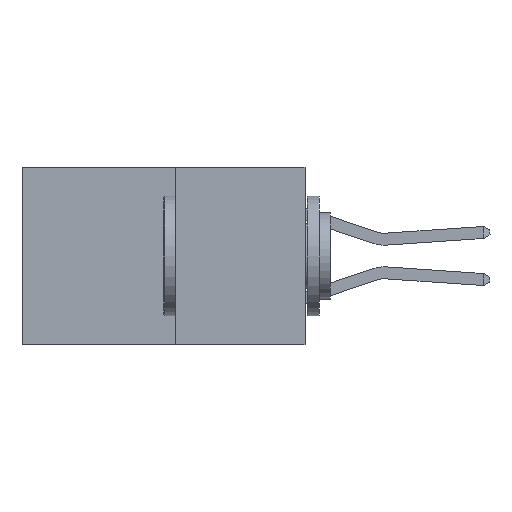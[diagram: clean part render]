
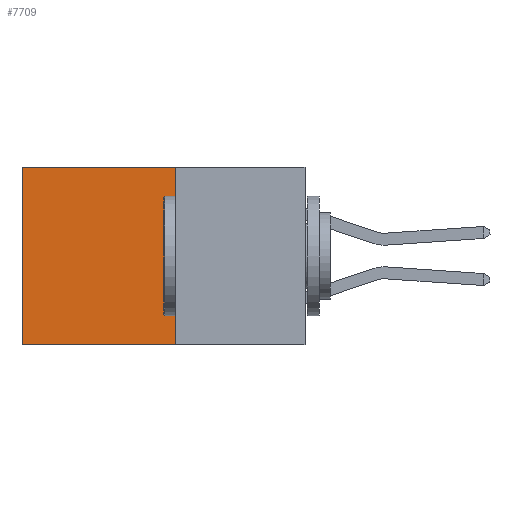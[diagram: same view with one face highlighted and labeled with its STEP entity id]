
A CAD part, left-side view. The second image highlights one B-rep face of the part: STEP entity #7709.
In plain terms, the highlighted planar face has unit normal (-1, 0, 0).
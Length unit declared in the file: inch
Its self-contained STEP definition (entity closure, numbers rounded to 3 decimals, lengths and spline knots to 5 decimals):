
#65 = CARTESIAN_POINT ( 'NONE',  ( 0.277, 0.27, 0. ) ) ;
#237 = VECTOR ( 'NONE', #8344, 39.37008 ) ;
#257 = EDGE_CURVE ( 'NONE', #1255, #6947, #2991, .T. ) ;
#728 = EDGE_CURVE ( 'NONE', #9189, #6947, #5139, .T. ) ;
#938 = DIRECTION ( 'NONE',  ( 0., 1., 0. ) ) ;
#1255 = VERTEX_POINT ( 'NONE', #4442 ) ;
#1571 = ORIENTED_EDGE ( 'NONE', *, *, #3591, .F. ) ;
#1621 = CARTESIAN_POINT ( 'NONE',  ( 0.277, 0.59, -0.37 ) ) ;
#1631 = AXIS2_PLACEMENT_3D ( 'NONE', #5844, #7537, #2435 ) ;
#1643 = CARTESIAN_POINT ( 'NONE',  ( 0.277, 0.27, -0.37 ) ) ;
#2001 = CARTESIAN_POINT ( 'NONE',  ( 0.277, 0.27, 0. ) ) ;
#2435 = DIRECTION ( 'NONE',  ( 0., 0., -1. ) ) ;
#2991 = LINE ( 'NONE', #8247, #7228 ) ;
#3591 = EDGE_CURVE ( 'NONE', #4736, #9189, #7426, .T. ) ;
#4192 = LINE ( 'NONE', #65, #5909 ) ;
#4442 = CARTESIAN_POINT ( 'NONE',  ( 0.277, 0.59, 0. ) ) ;
#4736 = VERTEX_POINT ( 'NONE', #2001 ) ;
#5139 = LINE ( 'NONE', #1643, #9230 ) ;
#5745 = ORIENTED_EDGE ( 'NONE', *, *, #257, .T. ) ;
#5844 = CARTESIAN_POINT ( 'NONE',  ( 0.277, 0.27, -0.37 ) ) ;
#5909 = VECTOR ( 'NONE', #6435, 39.37008 ) ;
#6435 = DIRECTION ( 'NONE',  ( 0., 1., 0. ) ) ;
#6946 = DIRECTION ( 'NONE',  ( 0., 0., -1. ) ) ;
#6947 = VERTEX_POINT ( 'NONE', #1621 ) ;
#7228 = VECTOR ( 'NONE', #6946, 39.37008 ) ;
#7426 = LINE ( 'NONE', #8457, #237 ) ;
#7440 = ORIENTED_EDGE ( 'NONE', *, *, #728, .F. ) ;
#7537 = DIRECTION ( 'NONE',  ( 1., 0., 0. ) ) ;
#7709 = ADVANCED_FACE ( 'NONE', ( #8164 ), #8333, .F. ) ;
#8164 = FACE_OUTER_BOUND ( 'NONE', #8541, .T. ) ;
#8247 = CARTESIAN_POINT ( 'NONE',  ( 0.277, 0.59, -0.37 ) ) ;
#8333 = PLANE ( 'NONE',  #1631 ) ;
#8344 = DIRECTION ( 'NONE',  ( 0., 0., -1. ) ) ;
#8457 = CARTESIAN_POINT ( 'NONE',  ( 0.277, 0.27, -0.37 ) ) ;
#8541 = EDGE_LOOP ( 'NONE', ( #5745, #7440, #1571, #10119 ) ) ;
#9189 = VERTEX_POINT ( 'NONE', #11011 ) ;
#9230 = VECTOR ( 'NONE', #938, 39.37008 ) ;
#9329 = EDGE_CURVE ( 'NONE', #4736, #1255, #4192, .T. ) ;
#10119 = ORIENTED_EDGE ( 'NONE', *, *, #9329, .T. ) ;
#11011 = CARTESIAN_POINT ( 'NONE',  ( 0.277, 0.27, -0.37 ) ) ;
